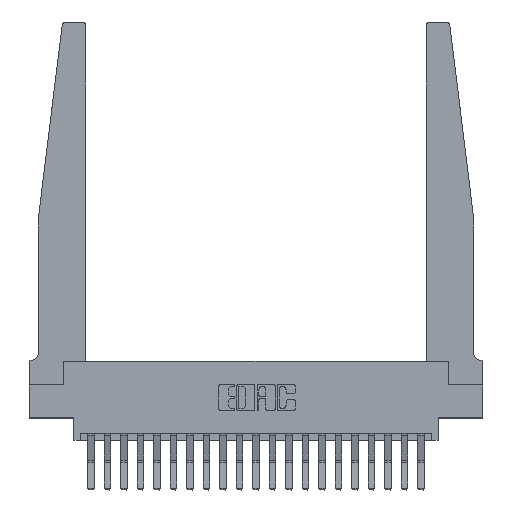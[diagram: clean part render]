
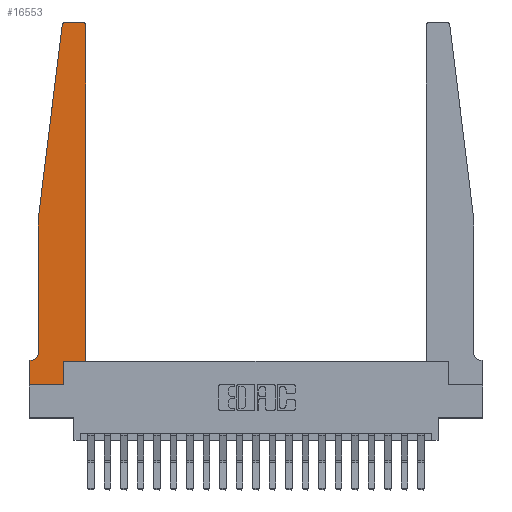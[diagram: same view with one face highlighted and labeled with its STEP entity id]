
A CAD part, top view. The second image highlights one B-rep face of the part: STEP entity #16553.
In plain terms, the highlighted planar face has unit normal (0, 0, 1).
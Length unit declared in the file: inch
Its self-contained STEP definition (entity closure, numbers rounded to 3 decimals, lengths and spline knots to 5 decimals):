
#211 = DIRECTION ( 'NONE',  ( 0., 0., 1. ) ) ;
#319 = EDGE_CURVE ( 'NONE', #21740, #13466, #9534, .T. ) ;
#406 = CARTESIAN_POINT ( 'NONE',  ( 0., 0., 0.37 ) ) ;
#673 = VERTEX_POINT ( 'NONE', #891 ) ;
#729 = ORIENTED_EDGE ( 'NONE', *, *, #20066, .T. ) ;
#811 = VECTOR ( 'NONE', #2350, 39.37008 ) ;
#891 = CARTESIAN_POINT ( 'NONE',  ( 0.2605, 0.18, 0.37 ) ) ;
#1307 = VERTEX_POINT ( 'NONE', #7538 ) ;
#1378 = CARTESIAN_POINT ( 'NONE',  ( 0.065, 1.25, 0.37 ) ) ;
#1558 = CARTESIAN_POINT ( 'NONE',  ( 0.015, 0.1875, 0.37 ) ) ;
#1739 = AXIS2_PLACEMENT_3D ( 'NONE', #15070, #211, #15629 ) ;
#2056 = CARTESIAN_POINT ( 'NONE',  ( 0.24675, 2.72367, 0.37 ) ) ;
#2350 = DIRECTION ( 'NONE',  ( -1., 0., 0. ) ) ;
#2581 = DIRECTION ( 'NONE',  ( 0., 0., -1. ) ) ;
#2789 = DIRECTION ( 'NONE',  ( -1., 0., 0. ) ) ;
#2868 = VERTEX_POINT ( 'NONE', #19472 ) ;
#3128 = AXIS2_PLACEMENT_3D ( 'NONE', #17816, #2581, #2789 ) ;
#3222 = DIRECTION ( 'NONE',  ( 0., 1., 0. ) ) ;
#3251 = EDGE_CURVE ( 'NONE', #7820, #5062, #13013, .T. ) ;
#3280 = CARTESIAN_POINT ( 'NONE',  ( 0.425, 0.18, 0.37 ) ) ;
#3473 = ORIENTED_EDGE ( 'NONE', *, *, #15901, .T. ) ;
#4173 = ORIENTED_EDGE ( 'NONE', *, *, #11393, .T. ) ;
#4420 = ORIENTED_EDGE ( 'NONE', *, *, #14144, .T. ) ;
#4512 = ORIENTED_EDGE ( 'NONE', *, *, #7577, .T. ) ;
#4918 = VECTOR ( 'NONE', #8159, 39.37008 ) ;
#4993 = CARTESIAN_POINT ( 'NONE',  ( 0.27653, 2.75, 0.37 ) ) ;
#5006 = LINE ( 'NONE', #18464, #17197 ) ;
#5048 = VERTEX_POINT ( 'NONE', #20583 ) ;
#5062 = VERTEX_POINT ( 'NONE', #1558 ) ;
#5112 = FACE_OUTER_BOUND ( 'NONE', #5114, .T. ) ;
#5114 = EDGE_LOOP ( 'NONE', ( #21729, #20453, #729, #3473, #16085, #20326, #17869, #4420, #4512, #12643, #4173, #6006 ) ) ;
#5345 = DIRECTION ( 'NONE',  ( 0., 0., 1. ) ) ;
#5671 = VECTOR ( 'NONE', #9935, 39.37008 ) ;
#5838 = CARTESIAN_POINT ( 'NONE',  ( 0.065, 1.25, 0.37 ) ) ;
#6006 = ORIENTED_EDGE ( 'NONE', *, *, #15413, .T. ) ;
#6015 = VERTEX_POINT ( 'NONE', #7657 ) ;
#6263 = LINE ( 'NONE', #16133, #9433 ) ;
#6527 = LINE ( 'NONE', #11143, #5671 ) ;
#6667 = EDGE_CURVE ( 'NONE', #5062, #2868, #6527, .T. ) ;
#7538 = CARTESIAN_POINT ( 'NONE',  ( 0.065, 1.25, 0.37 ) ) ;
#7577 = EDGE_CURVE ( 'NONE', #17300, #673, #5006, .T. ) ;
#7657 = CARTESIAN_POINT ( 'NONE',  ( 0., 0., 0.37 ) ) ;
#7820 = VERTEX_POINT ( 'NONE', #21258 ) ;
#7887 = CARTESIAN_POINT ( 'NONE',  ( 0.25, 2.75, 0.37 ) ) ;
#8114 = DIRECTION ( 'NONE',  ( 0., -1., 0. ) ) ;
#8159 = DIRECTION ( 'NONE',  ( 0., 1., 0. ) ) ;
#8623 = CARTESIAN_POINT ( 'NONE',  ( 0., 0.1875, 0.37 ) ) ;
#8730 = AXIS2_PLACEMENT_3D ( 'NONE', #8623, #5345, #18898 ) ;
#8911 = LINE ( 'NONE', #5838, #15493 ) ;
#9433 = VECTOR ( 'NONE', #21508, 39.37008 ) ;
#9534 = LINE ( 'NONE', #7887, #811 ) ;
#9935 = DIRECTION ( 'NONE',  ( -1., 0., 0. ) ) ;
#10249 = DIRECTION ( 'NONE',  ( 1., 0., 0. ) ) ;
#10376 = CIRCLE ( 'NONE', #16082, 0.03 ) ;
#10761 = VECTOR ( 'NONE', #8114, 39.37008 ) ;
#11143 = CARTESIAN_POINT ( 'NONE',  ( 0.065, 0.1875, 0.37 ) ) ;
#11393 = EDGE_CURVE ( 'NONE', #18802, #5048, #14506, .T. ) ;
#11604 = VERTEX_POINT ( 'NONE', #2056 ) ;
#11842 = PLANE ( 'NONE',  #8730 ) ;
#12136 = LINE ( 'NONE', #406, #14628 ) ;
#12335 = CIRCLE ( 'NONE', #1739, 0.03 ) ;
#12643 = ORIENTED_EDGE ( 'NONE', *, *, #19118, .T. ) ;
#12801 = CARTESIAN_POINT ( 'NONE',  ( 0.425, 0.18, 0.37 ) ) ;
#12961 = EDGE_CURVE ( 'NONE', #2868, #6015, #16118, .T. ) ;
#13013 = CIRCLE ( 'NONE', #3128, 0.05 ) ;
#13227 = CARTESIAN_POINT ( 'NONE',  ( 0.395, 2.72, 0.37 ) ) ;
#13335 = DIRECTION ( 'NONE',  ( 0., 0., 1. ) ) ;
#13466 = VERTEX_POINT ( 'NONE', #4993 ) ;
#14144 = EDGE_CURVE ( 'NONE', #6015, #17300, #12136, .T. ) ;
#14366 = DIRECTION ( 'NONE',  ( -0.122, -0.992, 0. ) ) ;
#14506 = LINE ( 'NONE', #12801, #4918 ) ;
#14628 = VECTOR ( 'NONE', #10249, 39.37008 ) ;
#15070 = CARTESIAN_POINT ( 'NONE',  ( 0.27653, 2.72, 0.37 ) ) ;
#15131 = CARTESIAN_POINT ( 'NONE',  ( 0.2605, 0., 0.37 ) ) ;
#15413 = EDGE_CURVE ( 'NONE', #5048, #21740, #10376, .T. ) ;
#15493 = VECTOR ( 'NONE', #14366, 39.37008 ) ;
#15629 = DIRECTION ( 'NONE',  ( 1., 0., 0. ) ) ;
#15901 = EDGE_CURVE ( 'NONE', #1307, #7820, #16665, .T. ) ;
#16082 = AXIS2_PLACEMENT_3D ( 'NONE', #13227, #13335, #16473 ) ;
#16085 = ORIENTED_EDGE ( 'NONE', *, *, #3251, .T. ) ;
#16118 = LINE ( 'NONE', #21493, #17796 ) ;
#16133 = CARTESIAN_POINT ( 'NONE',  ( 0.425, 0.18, 0.37 ) ) ;
#16473 = DIRECTION ( 'NONE',  ( 1., 0., 0. ) ) ;
#16553 = ADVANCED_FACE ( 'NONE', ( #5112 ), #11842, .T. ) ;
#16665 = LINE ( 'NONE', #1378, #10761 ) ;
#17197 = VECTOR ( 'NONE', #3222, 39.37008 ) ;
#17300 = VERTEX_POINT ( 'NONE', #15131 ) ;
#17796 = VECTOR ( 'NONE', #19845, 39.37008 ) ;
#17816 = CARTESIAN_POINT ( 'NONE',  ( 0.015, 0.2375, 0.37 ) ) ;
#17869 = ORIENTED_EDGE ( 'NONE', *, *, #12961, .T. ) ;
#18464 = CARTESIAN_POINT ( 'NONE',  ( 0.2605, 0.18, 0.37 ) ) ;
#18802 = VERTEX_POINT ( 'NONE', #3280 ) ;
#18898 = DIRECTION ( 'NONE',  ( 1., 0., 0. ) ) ;
#19118 = EDGE_CURVE ( 'NONE', #673, #18802, #6263, .T. ) ;
#19472 = CARTESIAN_POINT ( 'NONE',  ( 0., 0.1875, 0.37 ) ) ;
#19845 = DIRECTION ( 'NONE',  ( 0., -1., 0. ) ) ;
#20066 = EDGE_CURVE ( 'NONE', #11604, #1307, #8911, .T. ) ;
#20326 = ORIENTED_EDGE ( 'NONE', *, *, #6667, .T. ) ;
#20453 = ORIENTED_EDGE ( 'NONE', *, *, #21174, .T. ) ;
#20583 = CARTESIAN_POINT ( 'NONE',  ( 0.425, 2.72, 0.37 ) ) ;
#21174 = EDGE_CURVE ( 'NONE', #13466, #11604, #12335, .T. ) ;
#21258 = CARTESIAN_POINT ( 'NONE',  ( 0.065, 0.2375, 0.37 ) ) ;
#21493 = CARTESIAN_POINT ( 'NONE',  ( 0., 0., 0.37 ) ) ;
#21508 = DIRECTION ( 'NONE',  ( 1., 0., 0. ) ) ;
#21632 = CARTESIAN_POINT ( 'NONE',  ( 0.395, 2.75, 0.37 ) ) ;
#21729 = ORIENTED_EDGE ( 'NONE', *, *, #319, .T. ) ;
#21740 = VERTEX_POINT ( 'NONE', #21632 ) ;
